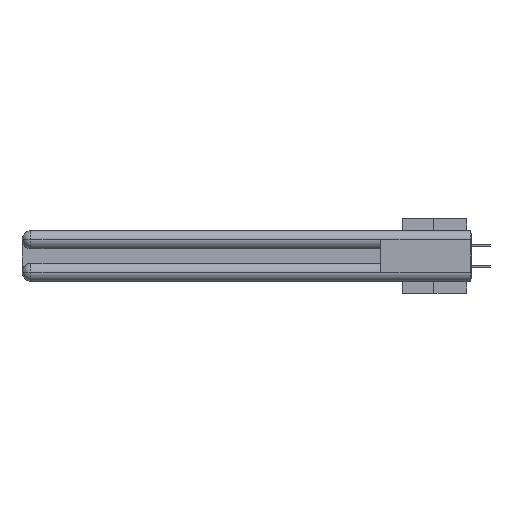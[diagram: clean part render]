
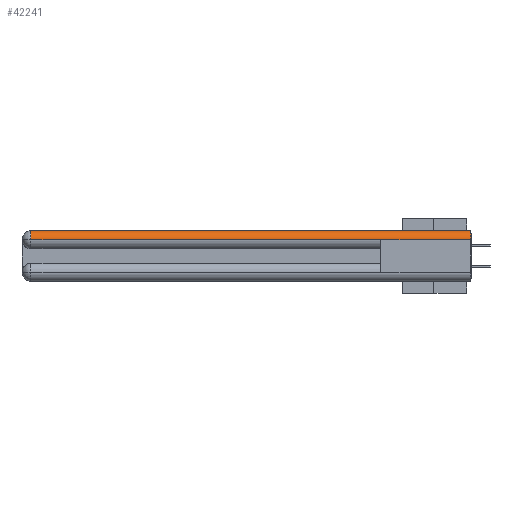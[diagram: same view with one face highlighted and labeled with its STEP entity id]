
A CAD part, left-side view. The second image highlights one B-rep face of the part: STEP entity #42241.
In plain terms, the highlighted cylindrical face has radius 1.562 mm (diameter 3.124 mm), a partial arc.
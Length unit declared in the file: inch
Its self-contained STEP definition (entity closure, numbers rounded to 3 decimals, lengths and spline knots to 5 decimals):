
#865 = VERTEX_POINT ( 'NONE', #41978 ) ;
#886 = DIRECTION ( 'NONE',  ( 0., -1., 0. ) ) ;
#1687 = DIRECTION ( 'NONE',  ( 0., -1., 0. ) ) ;
#2164 = EDGE_LOOP ( 'NONE', ( #26022, #18691, #17589, #24295, #34739 ) ) ;
#5090 = EDGE_CURVE ( 'NONE', #23151, #44690, #27299, .T. ) ;
#5823 = CARTESIAN_POINT ( 'NONE',  ( 0., 0.6, -0.0615 ) ) ;
#6795 = VECTOR ( 'NONE', #11758, 39.37008 ) ;
#8060 = CYLINDRICAL_SURFACE ( 'NONE', #16633, 0.0615 ) ;
#9283 = CARTESIAN_POINT ( 'NONE',  ( 0.0615, 0., 0. ) ) ;
#9433 = CARTESIAN_POINT ( 'NONE',  ( 0., 3., -0.0615 ) ) ;
#9538 = VERTEX_POINT ( 'NONE', #28784 ) ;
#11758 = DIRECTION ( 'NONE',  ( 0., -1., 0. ) ) ;
#16542 = EDGE_CURVE ( 'NONE', #44690, #28822, #45025, .T. ) ;
#16633 = AXIS2_PLACEMENT_3D ( 'NONE', #30053, #44933, #34282 ) ;
#17589 = ORIENTED_EDGE ( 'NONE', *, *, #16542, .T. ) ;
#18691 = ORIENTED_EDGE ( 'NONE', *, *, #5090, .T. ) ;
#18871 = LINE ( 'NONE', #9433, #27583 ) ;
#20286 = EDGE_CURVE ( 'NONE', #865, #28822, #18871, .T. ) ;
#23051 = CARTESIAN_POINT ( 'NONE',  ( 0.0615, 0., -0.0615 ) ) ;
#23151 = VERTEX_POINT ( 'NONE', #44811 ) ;
#23854 = CARTESIAN_POINT ( 'NONE',  ( 0.0615, 2.94, -0.0615 ) ) ;
#24294 = FACE_OUTER_BOUND ( 'NONE', #2164, .T. ) ;
#24295 = ORIENTED_EDGE ( 'NONE', *, *, #20286, .F. ) ;
#24633 = AXIS2_PLACEMENT_3D ( 'NONE', #23051, #886, #45747 ) ;
#26022 = ORIENTED_EDGE ( 'NONE', *, *, #47717, .F. ) ;
#26683 = CARTESIAN_POINT ( 'NONE',  ( 0., 3., -0.0615 ) ) ;
#27299 = CIRCLE ( 'NONE', #47123, 0.0615 ) ;
#27583 = VECTOR ( 'NONE', #38829, 39.37008 ) ;
#27597 = DIRECTION ( 'NONE',  ( 0., 0., 1. ) ) ;
#28784 = CARTESIAN_POINT ( 'NONE',  ( 0.0615, 0., 0. ) ) ;
#28822 = VERTEX_POINT ( 'NONE', #5823 ) ;
#30053 = CARTESIAN_POINT ( 'NONE',  ( 0.0615, 0., -0.0615 ) ) ;
#30812 = CIRCLE ( 'NONE', #24633, 0.0615 ) ;
#31526 = CARTESIAN_POINT ( 'NONE',  ( 0., 2.94, -0.0615 ) ) ;
#34282 = DIRECTION ( 'NONE',  ( 0., 0., 1. ) ) ;
#34739 = ORIENTED_EDGE ( 'NONE', *, *, #41297, .F. ) ;
#37739 = VECTOR ( 'NONE', #46566, 39.37008 ) ;
#38829 = DIRECTION ( 'NONE',  ( 0., 1., 0. ) ) ;
#41297 = EDGE_CURVE ( 'NONE', #9538, #865, #30812, .T. ) ;
#41978 = CARTESIAN_POINT ( 'NONE',  ( 0., 0., -0.0615 ) ) ;
#42241 = ADVANCED_FACE ( 'NONE', ( #24294 ), #8060, .T. ) ;
#44690 = VERTEX_POINT ( 'NONE', #31526 ) ;
#44811 = CARTESIAN_POINT ( 'NONE',  ( 0.0615, 2.94, 0. ) ) ;
#44933 = DIRECTION ( 'NONE',  ( 0., 1., 0. ) ) ;
#45025 = LINE ( 'NONE', #26683, #6795 ) ;
#45747 = DIRECTION ( 'NONE',  ( 1., 0., 0. ) ) ;
#46566 = DIRECTION ( 'NONE',  ( 0., -1., 0. ) ) ;
#47123 = AXIS2_PLACEMENT_3D ( 'NONE', #23854, #1687, #27597 ) ;
#47564 = LINE ( 'NONE', #9283, #37739 ) ;
#47717 = EDGE_CURVE ( 'NONE', #23151, #9538, #47564, .T. ) ;
